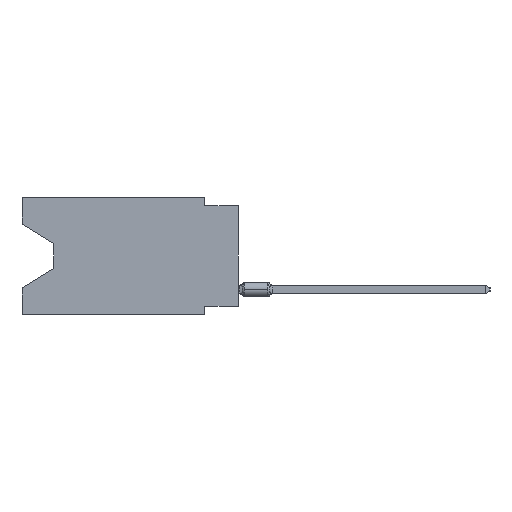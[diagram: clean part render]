
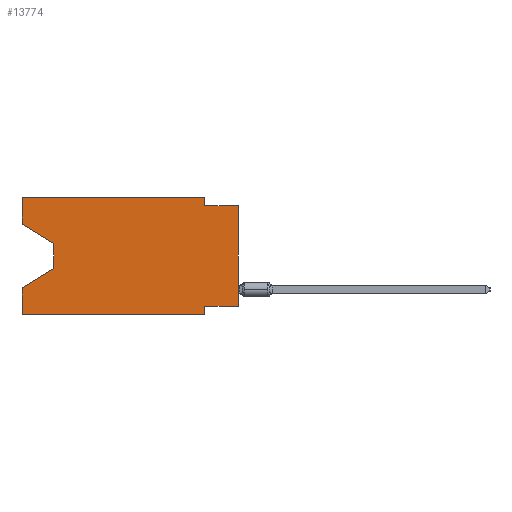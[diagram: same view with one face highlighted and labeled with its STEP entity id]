
A CAD part, left-side view. The second image highlights one B-rep face of the part: STEP entity #13774.
In plain terms, the highlighted planar face has unit normal (-1, 0, 0).
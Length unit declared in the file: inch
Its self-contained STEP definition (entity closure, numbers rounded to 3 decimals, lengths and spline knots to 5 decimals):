
#71 = VECTOR ( 'NONE', #46087, 39.37008 ) ;
#811 = PLANE ( 'NONE',  #36497 ) ;
#1293 = DIRECTION ( 'NONE',  ( 0., 1., 0. ) ) ;
#1786 = VERTEX_POINT ( 'NONE', #13502 ) ;
#3341 = ORIENTED_EDGE ( 'NONE', *, *, #20161, .T. ) ;
#5488 = CARTESIAN_POINT ( 'NONE',  ( 0., 0.645, 0. ) ) ;
#5661 = CARTESIAN_POINT ( 'NONE',  ( 0., 0.645, 0. ) ) ;
#5774 = LINE ( 'NONE', #5488, #40596 ) ;
#6165 = CARTESIAN_POINT ( 'NONE',  ( 0., 0.1, 0. ) ) ;
#6818 = VERTEX_POINT ( 'NONE', #20549 ) ;
#7969 = CARTESIAN_POINT ( 'NONE',  ( 0., 0., -0.025 ) ) ;
#8350 = DIRECTION ( 'NONE',  ( 0., -1., 0. ) ) ;
#9368 = LINE ( 'NONE', #37112, #10020 ) ;
#9938 = FACE_OUTER_BOUND ( 'NONE', #44617, .T. ) ;
#9972 = DIRECTION ( 'NONE',  ( 0., 0., 1. ) ) ;
#10020 = VECTOR ( 'NONE', #55098, 39.37008 ) ;
#10793 = ORIENTED_EDGE ( 'NONE', *, *, #11560, .F. ) ;
#11560 = EDGE_CURVE ( 'NONE', #43530, #31188, #46249, .T. ) ;
#13502 = CARTESIAN_POINT ( 'NONE',  ( 0., 0.645, -0.35 ) ) ;
#13774 = ADVANCED_FACE ( 'NONE', ( #9938 ), #811, .F. ) ;
#14111 = ORIENTED_EDGE ( 'NONE', *, *, #53015, .F. ) ;
#15349 = CARTESIAN_POINT ( 'NONE',  ( 0., 0., -0.325 ) ) ;
#17294 = EDGE_CURVE ( 'NONE', #26905, #17677, #38987, .T. ) ;
#17321 = CARTESIAN_POINT ( 'NONE',  ( 0., 0.55, -0.212 ) ) ;
#17521 = DIRECTION ( 'NONE',  ( 0., 0., -1. ) ) ;
#17677 = VERTEX_POINT ( 'NONE', #6165 ) ;
#17763 = CARTESIAN_POINT ( 'NONE',  ( 0., 0.645, -0.35 ) ) ;
#17894 = VECTOR ( 'NONE', #27257, 39.37008 ) ;
#18543 = VERTEX_POINT ( 'NONE', #29017 ) ;
#18782 = CARTESIAN_POINT ( 'NONE',  ( 0., 0.645, 0. ) ) ;
#19075 = DIRECTION ( 'NONE',  ( 0., 0., -1. ) ) ;
#20161 = EDGE_CURVE ( 'NONE', #22169, #6818, #39346, .T. ) ;
#20549 = CARTESIAN_POINT ( 'NONE',  ( 0., 0.55, -0.212 ) ) ;
#21192 = CARTESIAN_POINT ( 'NONE',  ( 0., 0.1, -0.35 ) ) ;
#22032 = LINE ( 'NONE', #17321, #56033 ) ;
#22138 = EDGE_CURVE ( 'NONE', #27144, #26905, #5774, .T. ) ;
#22169 = VERTEX_POINT ( 'NONE', #27580 ) ;
#23271 = CARTESIAN_POINT ( 'NONE',  ( 0., 0.645, -0.26975 ) ) ;
#23671 = EDGE_CURVE ( 'NONE', #18543, #34823, #26368, .T. ) ;
#23778 = VECTOR ( 'NONE', #1293, 39.37008 ) ;
#24863 = VECTOR ( 'NONE', #47415, 39.37008 ) ;
#25081 = CARTESIAN_POINT ( 'NONE',  ( 0., 0.645, 0. ) ) ;
#26021 = DIRECTION ( 'NONE',  ( 0., 0., -1. ) ) ;
#26368 = LINE ( 'NONE', #44417, #41648 ) ;
#26905 = VERTEX_POINT ( 'NONE', #48696 ) ;
#27144 = VERTEX_POINT ( 'NONE', #27387 ) ;
#27217 = ORIENTED_EDGE ( 'NONE', *, *, #23671, .F. ) ;
#27257 = DIRECTION ( 'NONE',  ( 0., -0.855, -0.519 ) ) ;
#27387 = CARTESIAN_POINT ( 'NONE',  ( 0., 0.645, -0.08025 ) ) ;
#27580 = CARTESIAN_POINT ( 'NONE',  ( 0., 0.55, -0.138 ) ) ;
#28060 = VECTOR ( 'NONE', #9972, 39.37008 ) ;
#28534 = CARTESIAN_POINT ( 'NONE',  ( 0., 0., 0. ) ) ;
#29017 = CARTESIAN_POINT ( 'NONE',  ( 0., 0.1, -0.325 ) ) ;
#29071 = EDGE_CURVE ( 'NONE', #45211, #18543, #36163, .T. ) ;
#29729 = LINE ( 'NONE', #45584, #17894 ) ;
#31188 = VERTEX_POINT ( 'NONE', #7969 ) ;
#31632 = EDGE_CURVE ( 'NONE', #6818, #32487, #22032, .T. ) ;
#32127 = VECTOR ( 'NONE', #26021, 39.37008 ) ;
#32487 = VERTEX_POINT ( 'NONE', #23271 ) ;
#34124 = EDGE_CURVE ( 'NONE', #1786, #34823, #58236, .T. ) ;
#34823 = VERTEX_POINT ( 'NONE', #21192 ) ;
#35195 = EDGE_CURVE ( 'NONE', #17677, #43530, #9368, .T. ) ;
#35917 = ORIENTED_EDGE ( 'NONE', *, *, #22138, .F. ) ;
#36163 = LINE ( 'NONE', #36736, #23778 ) ;
#36497 = AXIS2_PLACEMENT_3D ( 'NONE', #18782, #46247, #19075 ) ;
#36736 = CARTESIAN_POINT ( 'NONE',  ( 0., 0., -0.325 ) ) ;
#37112 = CARTESIAN_POINT ( 'NONE',  ( 0., 0.1, 0. ) ) ;
#37133 = LINE ( 'NONE', #28534, #28060 ) ;
#37491 = EDGE_CURVE ( 'NONE', #45211, #31188, #37133, .T. ) ;
#38107 = DIRECTION ( 'NONE',  ( 0., -1., 0. ) ) ;
#38494 = ORIENTED_EDGE ( 'NONE', *, *, #17294, .F. ) ;
#38987 = LINE ( 'NONE', #25081, #48095 ) ;
#39346 = LINE ( 'NONE', #58211, #32127 ) ;
#40119 = VECTOR ( 'NONE', #8350, 39.37008 ) ;
#40596 = VECTOR ( 'NONE', #45616, 39.37008 ) ;
#41089 = LINE ( 'NONE', #5661, #71 ) ;
#41648 = VECTOR ( 'NONE', #17521, 39.37008 ) ;
#43530 = VERTEX_POINT ( 'NONE', #56945 ) ;
#44417 = CARTESIAN_POINT ( 'NONE',  ( 0., 0.1, -0.35 ) ) ;
#44617 = EDGE_LOOP ( 'NONE', ( #49488, #3341, #44711, #14111, #49174, #27217, #44647, #52024, #10793, #52158, #38494, #35917 ) ) ;
#44647 = ORIENTED_EDGE ( 'NONE', *, *, #29071, .F. ) ;
#44711 = ORIENTED_EDGE ( 'NONE', *, *, #31632, .T. ) ;
#45211 = VERTEX_POINT ( 'NONE', #15349 ) ;
#45584 = CARTESIAN_POINT ( 'NONE',  ( 0., 0.645, -0.08025 ) ) ;
#45616 = DIRECTION ( 'NONE',  ( 0., 0., 1. ) ) ;
#46087 = DIRECTION ( 'NONE',  ( 0., 0., 1. ) ) ;
#46247 = DIRECTION ( 'NONE',  ( 1., 0., 0. ) ) ;
#46249 = LINE ( 'NONE', #47117, #24863 ) ;
#47117 = CARTESIAN_POINT ( 'NONE',  ( 0., 0., -0.025 ) ) ;
#47415 = DIRECTION ( 'NONE',  ( 0., -1., 0. ) ) ;
#48095 = VECTOR ( 'NONE', #38107, 39.37008 ) ;
#48696 = CARTESIAN_POINT ( 'NONE',  ( 0., 0.645, 0. ) ) ;
#49174 = ORIENTED_EDGE ( 'NONE', *, *, #34124, .T. ) ;
#49488 = ORIENTED_EDGE ( 'NONE', *, *, #52466, .T. ) ;
#52024 = ORIENTED_EDGE ( 'NONE', *, *, #37491, .T. ) ;
#52158 = ORIENTED_EDGE ( 'NONE', *, *, #35195, .F. ) ;
#52466 = EDGE_CURVE ( 'NONE', #27144, #22169, #29729, .T. ) ;
#53015 = EDGE_CURVE ( 'NONE', #1786, #32487, #41089, .T. ) ;
#53343 = DIRECTION ( 'NONE',  ( 0., 0.855, -0.519 ) ) ;
#55098 = DIRECTION ( 'NONE',  ( 0., 0., -1. ) ) ;
#56033 = VECTOR ( 'NONE', #53343, 39.37008 ) ;
#56945 = CARTESIAN_POINT ( 'NONE',  ( 0., 0.1, -0.025 ) ) ;
#58211 = CARTESIAN_POINT ( 'NONE',  ( 0., 0.55, -0.138 ) ) ;
#58236 = LINE ( 'NONE', #17763, #40119 ) ;
